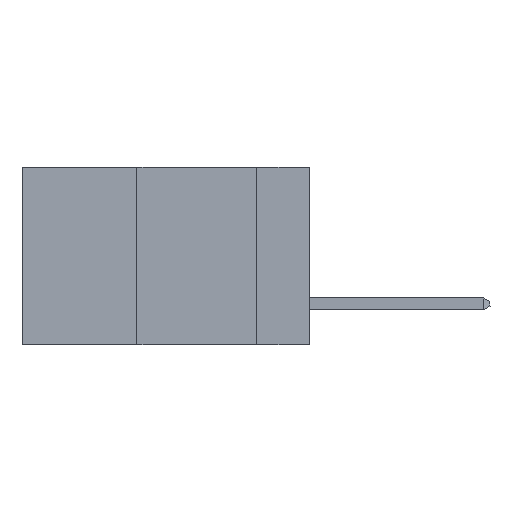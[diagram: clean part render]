
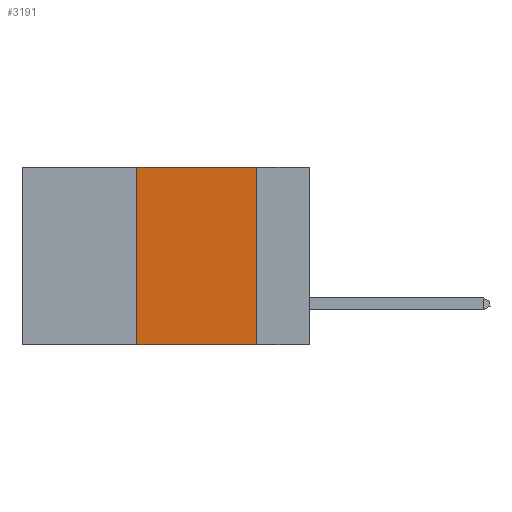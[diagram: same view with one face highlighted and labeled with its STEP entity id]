
A CAD part, left-side view. The second image highlights one B-rep face of the part: STEP entity #3191.
In plain terms, the highlighted planar face has unit normal (-1, 0, 0).
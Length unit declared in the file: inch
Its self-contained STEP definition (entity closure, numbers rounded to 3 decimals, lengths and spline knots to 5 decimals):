
#597 = ORIENTED_EDGE ( 'NONE', *, *, #8418, .F. ) ;
#693 = PLANE ( 'NONE',  #9417 ) ;
#810 = DIRECTION ( 'NONE',  ( 1., 0., 0. ) ) ;
#854 = CARTESIAN_POINT ( 'NONE',  ( 0., 0.36, 0. ) ) ;
#1179 = DIRECTION ( 'NONE',  ( 0., 0., -1. ) ) ;
#1980 = DIRECTION ( 'NONE',  ( 0., 0., 1. ) ) ;
#2362 = LINE ( 'NONE', #4961, #13283 ) ;
#3191 = ADVANCED_FACE ( 'NONE', ( #12095 ), #693, .F. ) ;
#3224 = DIRECTION ( 'NONE',  ( 0., 0., -1. ) ) ;
#3346 = VECTOR ( 'NONE', #6210, 39.37008 ) ;
#4151 = ORIENTED_EDGE ( 'NONE', *, *, #9125, .F. ) ;
#4548 = VERTEX_POINT ( 'NONE', #15072 ) ;
#4726 = EDGE_LOOP ( 'NONE', ( #12970, #4151, #597, #11279 ) ) ;
#4961 = CARTESIAN_POINT ( 'NONE',  ( 0., 0.11, 0. ) ) ;
#5511 = EDGE_CURVE ( 'NONE', #4548, #6391, #8830, .T. ) ;
#6210 = DIRECTION ( 'NONE',  ( 0., -1., 0. ) ) ;
#6391 = VERTEX_POINT ( 'NONE', #12986 ) ;
#6580 = CARTESIAN_POINT ( 'NONE',  ( 0., 0.36, 0. ) ) ;
#7061 = VECTOR ( 'NONE', #11019, 39.37008 ) ;
#8418 = EDGE_CURVE ( 'NONE', #4548, #10612, #8486, .T. ) ;
#8486 = LINE ( 'NONE', #854, #16277 ) ;
#8787 = CARTESIAN_POINT ( 'NONE',  ( 0., 0.6, 0. ) ) ;
#8830 = LINE ( 'NONE', #10004, #7061 ) ;
#9125 = EDGE_CURVE ( 'NONE', #10612, #11756, #10413, .T. ) ;
#9417 = AXIS2_PLACEMENT_3D ( 'NONE', #10713, #810, #3224 ) ;
#10004 = CARTESIAN_POINT ( 'NONE',  ( 0., 0.6, -0.37 ) ) ;
#10276 = CARTESIAN_POINT ( 'NONE',  ( 0., 0.11, 0. ) ) ;
#10413 = LINE ( 'NONE', #8787, #3346 ) ;
#10612 = VERTEX_POINT ( 'NONE', #6580 ) ;
#10713 = CARTESIAN_POINT ( 'NONE',  ( 0., 0.6, 0. ) ) ;
#11019 = DIRECTION ( 'NONE',  ( 0., -1., 0. ) ) ;
#11279 = ORIENTED_EDGE ( 'NONE', *, *, #5511, .T. ) ;
#11756 = VERTEX_POINT ( 'NONE', #10276 ) ;
#12095 = FACE_OUTER_BOUND ( 'NONE', #4726, .T. ) ;
#12970 = ORIENTED_EDGE ( 'NONE', *, *, #12973, .F. ) ;
#12973 = EDGE_CURVE ( 'NONE', #11756, #6391, #2362, .T. ) ;
#12986 = CARTESIAN_POINT ( 'NONE',  ( 0., 0.11, -0.37 ) ) ;
#13283 = VECTOR ( 'NONE', #1179, 39.37008 ) ;
#15072 = CARTESIAN_POINT ( 'NONE',  ( 0., 0.36, -0.37 ) ) ;
#16277 = VECTOR ( 'NONE', #1980, 39.37008 ) ;
